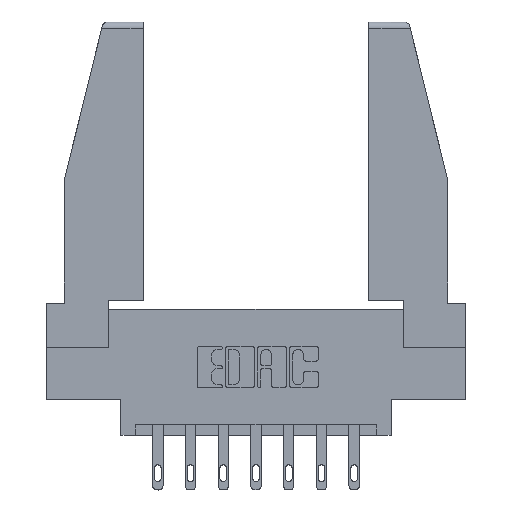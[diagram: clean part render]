
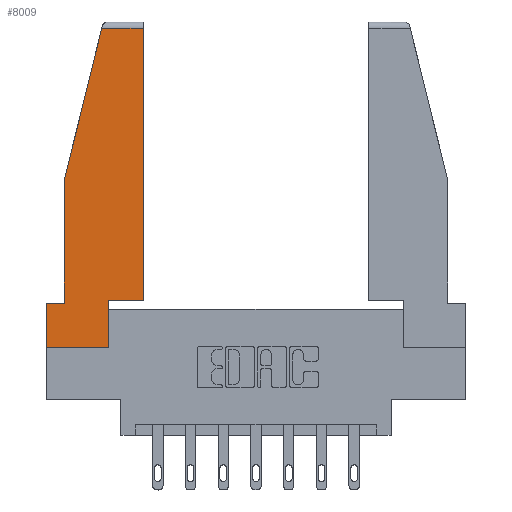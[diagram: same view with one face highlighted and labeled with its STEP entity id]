
A CAD part, top view. The second image highlights one B-rep face of the part: STEP entity #8009.
In plain terms, the highlighted planar face has unit normal (0, 0, 1).
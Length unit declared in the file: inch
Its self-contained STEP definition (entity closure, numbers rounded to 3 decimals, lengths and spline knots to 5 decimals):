
#298 = LINE ( 'NONE', #5314, #5130 ) ;
#521 = ORIENTED_EDGE ( 'NONE', *, *, #7398, .T. ) ;
#527 = LINE ( 'NONE', #7572, #8676 ) ;
#1355 = VERTEX_POINT ( 'NONE', #12036 ) ;
#1917 = CARTESIAN_POINT ( 'NONE',  ( 0., 0.21, 0. ) ) ;
#2102 = DIRECTION ( 'NONE',  ( -1., 0., 0. ) ) ;
#2285 = VECTOR ( 'NONE', #12135, 39.37008 ) ;
#2596 = EDGE_LOOP ( 'NONE', ( #6283, #3456, #521, #8468, #5003, #4751, #3992, #7939, #12243 ) ) ;
#2635 = DIRECTION ( 'NONE',  ( 0., -1., 0. ) ) ;
#2787 = VECTOR ( 'NONE', #4396, 39.37008 ) ;
#3061 = LINE ( 'NONE', #11141, #2285 ) ;
#3456 = ORIENTED_EDGE ( 'NONE', *, *, #6085, .T. ) ;
#3584 = VECTOR ( 'NONE', #12372, 39.37008 ) ;
#3639 = VERTEX_POINT ( 'NONE', #6453 ) ;
#3840 = VERTEX_POINT ( 'NONE', #5663 ) ;
#3930 = VERTEX_POINT ( 'NONE', #9531 ) ;
#3992 = ORIENTED_EDGE ( 'NONE', *, *, #8539, .T. ) ;
#4188 = LINE ( 'NONE', #4527, #3584 ) ;
#4396 = DIRECTION ( 'NONE',  ( 0., 1., 0. ) ) ;
#4399 = VERTEX_POINT ( 'NONE', #12079 ) ;
#4430 = EDGE_CURVE ( 'NONE', #3840, #3639, #4486, .T. ) ;
#4486 = LINE ( 'NONE', #1917, #8975 ) ;
#4527 = CARTESIAN_POINT ( 'NONE',  ( 0.271, 1.55, 0. ) ) ;
#4641 = CARTESIAN_POINT ( 'NONE',  ( 0.297, 0.223, 0. ) ) ;
#4751 = ORIENTED_EDGE ( 'NONE', *, *, #12033, .T. ) ;
#4777 = CARTESIAN_POINT ( 'NONE',  ( 0., 0., 0. ) ) ;
#4930 = LINE ( 'NONE', #8092, #9731 ) ;
#4988 = AXIS2_PLACEMENT_3D ( 'NONE', #7223, #5243, #10001 ) ;
#4991 = LINE ( 'NONE', #9184, #11011 ) ;
#5003 = ORIENTED_EDGE ( 'NONE', *, *, #4430, .T. ) ;
#5130 = VECTOR ( 'NONE', #2635, 39.37008 ) ;
#5198 = DIRECTION ( 'NONE',  ( -1., 0., 0. ) ) ;
#5243 = DIRECTION ( 'NONE',  ( 0., 0., 1. ) ) ;
#5314 = CARTESIAN_POINT ( 'NONE',  ( 0., 0.21, 0. ) ) ;
#5512 = CARTESIAN_POINT ( 'NONE',  ( 0., 0., 0. ) ) ;
#5663 = CARTESIAN_POINT ( 'NONE',  ( 0.086, 0.21, 0. ) ) ;
#5729 = CARTESIAN_POINT ( 'NONE',  ( 0.461, 1.52, 0. ) ) ;
#6085 = EDGE_CURVE ( 'NONE', #8187, #4399, #4991, .T. ) ;
#6283 = ORIENTED_EDGE ( 'NONE', *, *, #9306, .T. ) ;
#6453 = CARTESIAN_POINT ( 'NONE',  ( 0., 0.21, 0. ) ) ;
#6594 = LINE ( 'NONE', #4777, #10206 ) ;
#7089 = PLANE ( 'NONE',  #4988 ) ;
#7223 = CARTESIAN_POINT ( 'NONE',  ( 0., 0., 0. ) ) ;
#7240 = VERTEX_POINT ( 'NONE', #5512 ) ;
#7398 = EDGE_CURVE ( 'NONE', #4399, #3930, #4188, .T. ) ;
#7572 = CARTESIAN_POINT ( 'NONE',  ( 0.086, 0.8, 0. ) ) ;
#7675 = VERTEX_POINT ( 'NONE', #9232 ) ;
#7939 = ORIENTED_EDGE ( 'NONE', *, *, #8682, .T. ) ;
#8009 = ADVANCED_FACE ( 'NONE', ( #10816 ), #7089, .T. ) ;
#8092 = CARTESIAN_POINT ( 'NONE',  ( 0.297, 0., 0. ) ) ;
#8133 = EDGE_CURVE ( 'NONE', #3930, #3840, #527, .T. ) ;
#8136 = DIRECTION ( 'NONE',  ( 0., 1., 0. ) ) ;
#8187 = VERTEX_POINT ( 'NONE', #5729 ) ;
#8468 = ORIENTED_EDGE ( 'NONE', *, *, #8133, .T. ) ;
#8539 = EDGE_CURVE ( 'NONE', #7240, #7675, #6594, .T. ) ;
#8676 = VECTOR ( 'NONE', #9522, 39.37008 ) ;
#8682 = EDGE_CURVE ( 'NONE', #7675, #12483, #4930, .T. ) ;
#8975 = VECTOR ( 'NONE', #2102, 39.37008 ) ;
#9176 = CARTESIAN_POINT ( 'NONE',  ( 0.461, 0.223, 0. ) ) ;
#9184 = CARTESIAN_POINT ( 'NONE',  ( 0., 1.52, 0. ) ) ;
#9232 = CARTESIAN_POINT ( 'NONE',  ( 0.297, 0., 0. ) ) ;
#9306 = EDGE_CURVE ( 'NONE', #1355, #8187, #11083, .T. ) ;
#9522 = DIRECTION ( 'NONE',  ( 0., -1., 0. ) ) ;
#9531 = CARTESIAN_POINT ( 'NONE',  ( 0.086, 0.8, 0. ) ) ;
#9731 = VECTOR ( 'NONE', #8136, 39.37008 ) ;
#10001 = DIRECTION ( 'NONE',  ( 1., 0., 0. ) ) ;
#10206 = VECTOR ( 'NONE', #12273, 39.37008 ) ;
#10816 = FACE_OUTER_BOUND ( 'NONE', #2596, .T. ) ;
#10845 = EDGE_CURVE ( 'NONE', #12483, #1355, #3061, .T. ) ;
#11011 = VECTOR ( 'NONE', #5198, 39.37008 ) ;
#11083 = LINE ( 'NONE', #9176, #2787 ) ;
#11141 = CARTESIAN_POINT ( 'NONE',  ( 0.297, 0.223, 0. ) ) ;
#12033 = EDGE_CURVE ( 'NONE', #3639, #7240, #298, .T. ) ;
#12036 = CARTESIAN_POINT ( 'NONE',  ( 0.461, 0.223, 0. ) ) ;
#12079 = CARTESIAN_POINT ( 'NONE',  ( 0.2636, 1.52, 0. ) ) ;
#12135 = DIRECTION ( 'NONE',  ( 1., 0., 0. ) ) ;
#12243 = ORIENTED_EDGE ( 'NONE', *, *, #10845, .T. ) ;
#12273 = DIRECTION ( 'NONE',  ( 1., 0., 0. ) ) ;
#12372 = DIRECTION ( 'NONE',  ( -0.239, -0.971, 0. ) ) ;
#12483 = VERTEX_POINT ( 'NONE', #4641 ) ;
